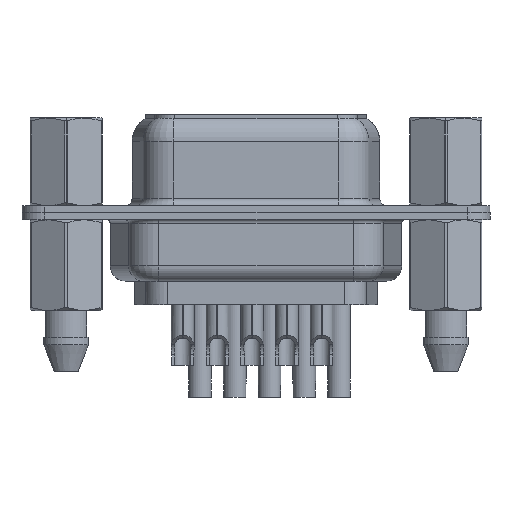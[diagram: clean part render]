
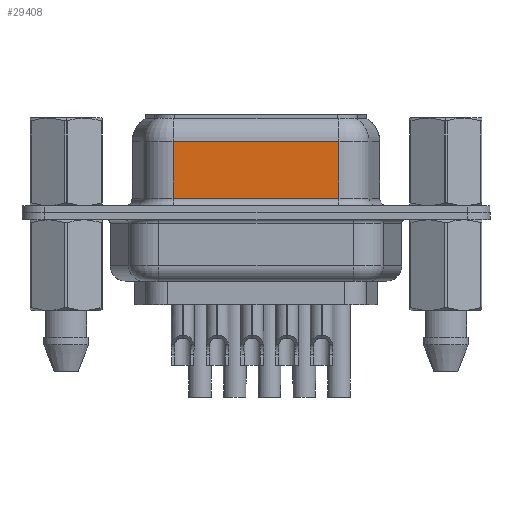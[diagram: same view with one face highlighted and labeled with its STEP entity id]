
A CAD part, front view. The second image highlights one B-rep face of the part: STEP entity #29408.
In plain terms, the highlighted planar face has unit normal (0, -1, 0).
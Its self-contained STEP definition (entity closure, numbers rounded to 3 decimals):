
#807 = ORIENTED_EDGE ( 'NONE', *, *, #27302, .T. ) ;
#2857 = CARTESIAN_POINT ( 'NONE',  ( 7.033, -3.95, 0.95 ) ) ;
#3259 = CARTESIAN_POINT ( 'NONE',  ( 17.957, -3.95, 4.7 ) ) ;
#3758 = EDGE_LOOP ( 'NONE', ( #22747, #28551, #11090, #807 ) ) ;
#3995 = AXIS2_PLACEMENT_3D ( 'NONE', #25157, #27509, #13398 ) ;
#5602 = VERTEX_POINT ( 'NONE', #2857 ) ;
#5695 = EDGE_CURVE ( 'NONE', #15406, #26033, #11390, .T. ) ;
#7186 = VECTOR ( 'NONE', #29427, 1000. ) ;
#7305 = LINE ( 'NONE', #25764, #25396 ) ;
#7754 = VECTOR ( 'NONE', #15124, 1000. ) ;
#7921 = FACE_OUTER_BOUND ( 'NONE', #3758, .T. ) ;
#11090 = ORIENTED_EDGE ( 'NONE', *, *, #24856, .T. ) ;
#11390 = LINE ( 'NONE', #12579, #29465 ) ;
#12579 = CARTESIAN_POINT ( 'NONE',  ( 17.957, -3.95, 6.45 ) ) ;
#12940 = CARTESIAN_POINT ( 'NONE',  ( 17.957, -3.95, 4.7 ) ) ;
#13398 = DIRECTION ( 'NONE',  ( 0., 0., 1. ) ) ;
#15124 = DIRECTION ( 'NONE',  ( 0., 0., -1. ) ) ;
#15406 = VERTEX_POINT ( 'NONE', #3259 ) ;
#15560 = LINE ( 'NONE', #29240, #7754 ) ;
#18791 = EDGE_CURVE ( 'NONE', #15406, #26076, #19038, .T. ) ;
#19038 = LINE ( 'NONE', #12940, #7186 ) ;
#20298 = PLANE ( 'NONE',  #3995 ) ;
#22020 = CARTESIAN_POINT ( 'NONE',  ( 7.033, -3.95, 4.7 ) ) ;
#22058 = DIRECTION ( 'NONE',  ( 0., 0., -1. ) ) ;
#22747 = ORIENTED_EDGE ( 'NONE', *, *, #5695, .F. ) ;
#24856 = EDGE_CURVE ( 'NONE', #26076, #5602, #15560, .T. ) ;
#25157 = CARTESIAN_POINT ( 'NONE',  ( 17.957, -3.95, 6.45 ) ) ;
#25396 = VECTOR ( 'NONE', #25873, 1000. ) ;
#25764 = CARTESIAN_POINT ( 'NONE',  ( 17.957, -3.95, 0.95 ) ) ;
#25873 = DIRECTION ( 'NONE',  ( 1., 0., 0. ) ) ;
#26033 = VERTEX_POINT ( 'NONE', #26357 ) ;
#26076 = VERTEX_POINT ( 'NONE', #22020 ) ;
#26357 = CARTESIAN_POINT ( 'NONE',  ( 17.957, -3.95, 0.95 ) ) ;
#27302 = EDGE_CURVE ( 'NONE', #5602, #26033, #7305, .T. ) ;
#27509 = DIRECTION ( 'NONE',  ( 0., 1., 0. ) ) ;
#28551 = ORIENTED_EDGE ( 'NONE', *, *, #18791, .T. ) ;
#29240 = CARTESIAN_POINT ( 'NONE',  ( 7.033, -3.95, 6.45 ) ) ;
#29408 = ADVANCED_FACE ( 'NONE', ( #7921 ), #20298, .F. ) ;
#29427 = DIRECTION ( 'NONE',  ( -1., 0., 0. ) ) ;
#29465 = VECTOR ( 'NONE', #22058, 1000. ) ;
